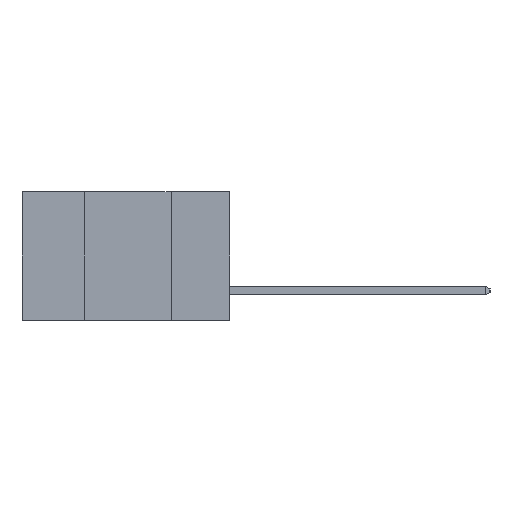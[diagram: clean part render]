
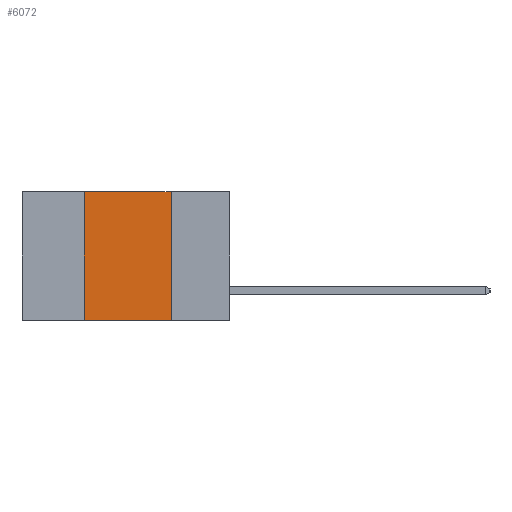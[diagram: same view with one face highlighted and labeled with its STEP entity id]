
A CAD part, left-side view. The second image highlights one B-rep face of the part: STEP entity #6072.
In plain terms, the highlighted planar face has unit normal (-1, 0, 0).
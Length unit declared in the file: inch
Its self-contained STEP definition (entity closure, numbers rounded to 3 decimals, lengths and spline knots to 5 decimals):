
#505 = LINE ( 'NONE', #5053, #10023 ) ;
#853 = FACE_OUTER_BOUND ( 'NONE', #8296, .T. ) ;
#1191 = EDGE_CURVE ( 'NONE', #4329, #6219, #505, .T. ) ;
#1603 = CARTESIAN_POINT ( 'NONE',  ( 0., 0.42, -0.37 ) ) ;
#2063 = VERTEX_POINT ( 'NONE', #9156 ) ;
#3523 = DIRECTION ( 'NONE',  ( 0., 0., -1. ) ) ;
#3528 = LINE ( 'NONE', #10249, #7946 ) ;
#3885 = VECTOR ( 'NONE', #7755, 39.37008 ) ;
#3916 = CARTESIAN_POINT ( 'NONE',  ( 0., 0.42, 0. ) ) ;
#4229 = DIRECTION ( 'NONE',  ( 0., -1., 0. ) ) ;
#4329 = VERTEX_POINT ( 'NONE', #1603 ) ;
#4359 = DIRECTION ( 'NONE',  ( 1., 0., 0. ) ) ;
#5053 = CARTESIAN_POINT ( 'NONE',  ( 0., 0.6, -0.37 ) ) ;
#5306 = AXIS2_PLACEMENT_3D ( 'NONE', #9441, #4359, #10215 ) ;
#6072 = ADVANCED_FACE ( 'NONE', ( #853 ), #7832, .F. ) ;
#6091 = EDGE_CURVE ( 'NONE', #4329, #8868, #3528, .T. ) ;
#6132 = DIRECTION ( 'NONE',  ( 0., 0., 1. ) ) ;
#6219 = VERTEX_POINT ( 'NONE', #11163 ) ;
#6558 = VECTOR ( 'NONE', #3523, 39.37008 ) ;
#7168 = ORIENTED_EDGE ( 'NONE', *, *, #6091, .F. ) ;
#7189 = ORIENTED_EDGE ( 'NONE', *, *, #1191, .T. ) ;
#7393 = LINE ( 'NONE', #11010, #6558 ) ;
#7587 = ORIENTED_EDGE ( 'NONE', *, *, #10496, .F. ) ;
#7671 = EDGE_CURVE ( 'NONE', #2063, #6219, #7393, .T. ) ;
#7687 = ORIENTED_EDGE ( 'NONE', *, *, #7671, .F. ) ;
#7755 = DIRECTION ( 'NONE',  ( 0., -1., 0. ) ) ;
#7832 = PLANE ( 'NONE',  #5306 ) ;
#7946 = VECTOR ( 'NONE', #6132, 39.37008 ) ;
#8296 = EDGE_LOOP ( 'NONE', ( #7687, #7587, #7168, #7189 ) ) ;
#8551 = CARTESIAN_POINT ( 'NONE',  ( 0., 0.6, 0. ) ) ;
#8868 = VERTEX_POINT ( 'NONE', #3916 ) ;
#9156 = CARTESIAN_POINT ( 'NONE',  ( 0., 0.17, 0. ) ) ;
#9441 = CARTESIAN_POINT ( 'NONE',  ( 0., 0.6, 0. ) ) ;
#10023 = VECTOR ( 'NONE', #4229, 39.37008 ) ;
#10215 = DIRECTION ( 'NONE',  ( 0., 0., -1. ) ) ;
#10249 = CARTESIAN_POINT ( 'NONE',  ( 0., 0.42, -0.37 ) ) ;
#10496 = EDGE_CURVE ( 'NONE', #8868, #2063, #10561, .T. ) ;
#10561 = LINE ( 'NONE', #8551, #3885 ) ;
#11010 = CARTESIAN_POINT ( 'NONE',  ( 0., 0.17, -0.37 ) ) ;
#11163 = CARTESIAN_POINT ( 'NONE',  ( 0., 0.17, -0.37 ) ) ;
